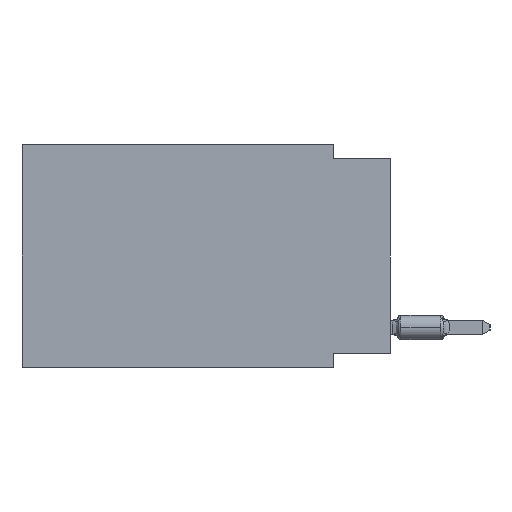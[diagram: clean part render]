
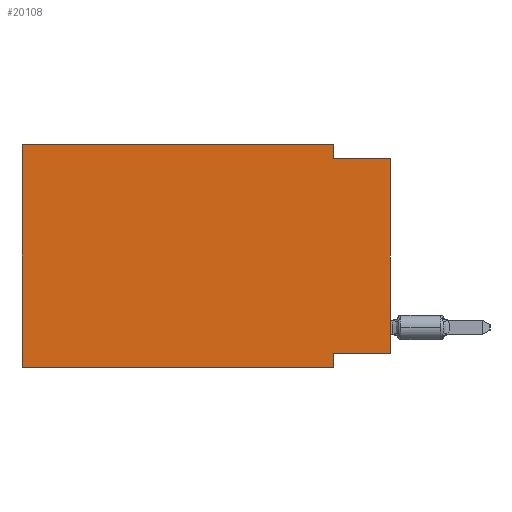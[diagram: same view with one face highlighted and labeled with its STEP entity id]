
A CAD part, left-side view. The second image highlights one B-rep face of the part: STEP entity #20108.
In plain terms, the highlighted planar face has unit normal (-1, 0, 0).
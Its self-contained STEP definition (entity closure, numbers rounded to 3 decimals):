
#4 = EDGE_CURVE ( 'NONE', #12438, #587, #23248, .T. ) ;
#587 = VERTEX_POINT ( 'NONE', #15640 ) ;
#670 = EDGE_LOOP ( 'NONE', ( #17681, #8311, #15870, #27073, #7670, #20170, #18608, #3346 ) ) ;
#1250 = CARTESIAN_POINT ( 'NONE',  ( 0., 0., 0. ) ) ;
#1723 = DIRECTION ( 'NONE',  ( 0., -1., 0. ) ) ;
#1953 = DIRECTION ( 'NONE',  ( 0., 0., -1. ) ) ;
#2282 = DIRECTION ( 'NONE',  ( 1., 0., 0. ) ) ;
#2652 = EDGE_CURVE ( 'NONE', #17486, #12241, #5818, .T. ) ;
#3346 = ORIENTED_EDGE ( 'NONE', *, *, #11278, .F. ) ;
#4166 = DIRECTION ( 'NONE',  ( 0., 0., -1. ) ) ;
#4242 = LINE ( 'NONE', #28380, #9116 ) ;
#4548 = DIRECTION ( 'NONE',  ( 0., 1., 0. ) ) ;
#4885 = VECTOR ( 'NONE', #7000, 1000. ) ;
#5818 = LINE ( 'NONE', #15590, #20924 ) ;
#5825 = EDGE_CURVE ( 'NONE', #12438, #13689, #28200, .T. ) ;
#6029 = VERTEX_POINT ( 'NONE', #9122 ) ;
#6677 = LINE ( 'NONE', #19031, #10885 ) ;
#7000 = DIRECTION ( 'NONE',  ( 0., -1., 0. ) ) ;
#7063 = CARTESIAN_POINT ( 'NONE',  ( 0., 2.54, -9.906 ) ) ;
#7190 = CARTESIAN_POINT ( 'NONE',  ( 0., 16.383, -9.906 ) ) ;
#7670 = ORIENTED_EDGE ( 'NONE', *, *, #4, .F. ) ;
#8311 = ORIENTED_EDGE ( 'NONE', *, *, #2652, .F. ) ;
#9116 = VECTOR ( 'NONE', #4548, 1000. ) ;
#9122 = CARTESIAN_POINT ( 'NONE',  ( 0., 0., -9.271 ) ) ;
#9675 = CARTESIAN_POINT ( 'NONE',  ( 0., 2.54, -9.906 ) ) ;
#10114 = CARTESIAN_POINT ( 'NONE',  ( 0., 2.54, -0.635 ) ) ;
#10474 = VECTOR ( 'NONE', #4166, 1000. ) ;
#10528 = VECTOR ( 'NONE', #20132, 1000. ) ;
#10885 = VECTOR ( 'NONE', #1723, 1000. ) ;
#11278 = EDGE_CURVE ( 'NONE', #6029, #17404, #4242, .T. ) ;
#12036 = EDGE_CURVE ( 'NONE', #17404, #13689, #28421, .T. ) ;
#12241 = VERTEX_POINT ( 'NONE', #26398 ) ;
#12438 = VERTEX_POINT ( 'NONE', #7190 ) ;
#13457 = CARTESIAN_POINT ( 'NONE',  ( 0., 2.54, 0. ) ) ;
#13660 = VECTOR ( 'NONE', #28204, 1000. ) ;
#13689 = VERTEX_POINT ( 'NONE', #9675 ) ;
#15482 = LINE ( 'NONE', #13457, #10474 ) ;
#15590 = CARTESIAN_POINT ( 'NONE',  ( 0., 0., -0.635 ) ) ;
#15640 = CARTESIAN_POINT ( 'NONE',  ( 0., 16.383, 0. ) ) ;
#15870 = ORIENTED_EDGE ( 'NONE', *, *, #23269, .F. ) ;
#15973 = LINE ( 'NONE', #1250, #10528 ) ;
#16064 = VECTOR ( 'NONE', #20817, 1000. ) ;
#16323 = CARTESIAN_POINT ( 'NONE',  ( 0., 2.54, -9.271 ) ) ;
#17404 = VERTEX_POINT ( 'NONE', #16323 ) ;
#17486 = VERTEX_POINT ( 'NONE', #10114 ) ;
#17681 = ORIENTED_EDGE ( 'NONE', *, *, #21272, .T. ) ;
#17713 = EDGE_CURVE ( 'NONE', #587, #26583, #6677, .T. ) ;
#17847 = AXIS2_PLACEMENT_3D ( 'NONE', #23169, #2282, #1953 ) ;
#18608 = ORIENTED_EDGE ( 'NONE', *, *, #12036, .F. ) ;
#19031 = CARTESIAN_POINT ( 'NONE',  ( 0., 16.383, 0. ) ) ;
#20108 = ADVANCED_FACE ( 'NONE', ( #21010 ), #24931, .F. ) ;
#20132 = DIRECTION ( 'NONE',  ( 0., 0., 1. ) ) ;
#20170 = ORIENTED_EDGE ( 'NONE', *, *, #5825, .T. ) ;
#20279 = CARTESIAN_POINT ( 'NONE',  ( 0., 2.54, 0. ) ) ;
#20817 = DIRECTION ( 'NONE',  ( 0., 0., -1. ) ) ;
#20924 = VECTOR ( 'NONE', #24688, 1000. ) ;
#21010 = FACE_OUTER_BOUND ( 'NONE', #670, .T. ) ;
#21272 = EDGE_CURVE ( 'NONE', #6029, #12241, #15973, .T. ) ;
#23169 = CARTESIAN_POINT ( 'NONE',  ( 0., 16.383, 0. ) ) ;
#23248 = LINE ( 'NONE', #25583, #13660 ) ;
#23269 = EDGE_CURVE ( 'NONE', #26583, #17486, #15482, .T. ) ;
#24688 = DIRECTION ( 'NONE',  ( 0., -1., 0. ) ) ;
#24931 = PLANE ( 'NONE',  #17847 ) ;
#25583 = CARTESIAN_POINT ( 'NONE',  ( 0., 16.383, 0. ) ) ;
#26398 = CARTESIAN_POINT ( 'NONE',  ( 0., 0., -0.635 ) ) ;
#26583 = VERTEX_POINT ( 'NONE', #20279 ) ;
#27073 = ORIENTED_EDGE ( 'NONE', *, *, #17713, .F. ) ;
#28200 = LINE ( 'NONE', #28514, #4885 ) ;
#28204 = DIRECTION ( 'NONE',  ( 0., 0., 1. ) ) ;
#28380 = CARTESIAN_POINT ( 'NONE',  ( 0., 0., -9.271 ) ) ;
#28421 = LINE ( 'NONE', #7063, #16064 ) ;
#28514 = CARTESIAN_POINT ( 'NONE',  ( 0., 16.383, -9.906 ) ) ;
